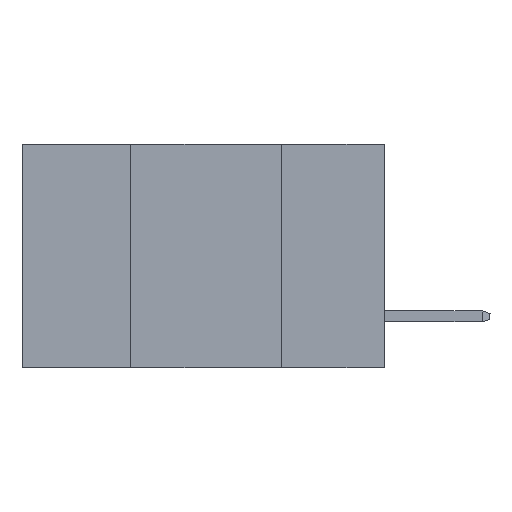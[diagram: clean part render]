
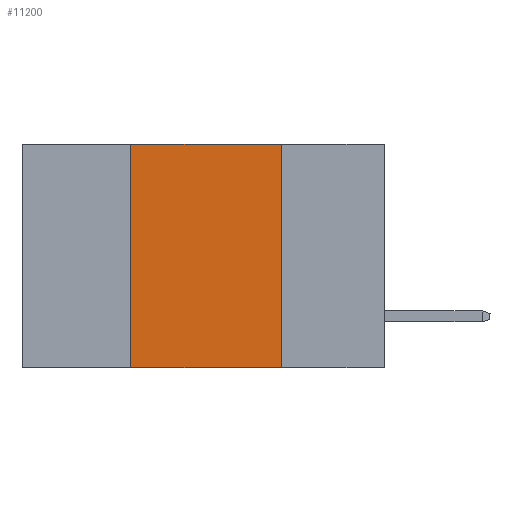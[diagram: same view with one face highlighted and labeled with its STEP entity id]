
A CAD part, left-side view. The second image highlights one B-rep face of the part: STEP entity #11200.
In plain terms, the highlighted planar face has unit normal (-1, 0, 0).
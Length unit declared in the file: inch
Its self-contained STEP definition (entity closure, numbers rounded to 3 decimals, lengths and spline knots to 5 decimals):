
#228 = FACE_OUTER_BOUND ( 'NONE', #8586, .T. ) ;
#1096 = VECTOR ( 'NONE', #9486, 39.37008 ) ;
#1423 = VECTOR ( 'NONE', #8526, 39.37008 ) ;
#1829 = ORIENTED_EDGE ( 'NONE', *, *, #15699, .F. ) ;
#1856 = EDGE_CURVE ( 'NONE', #16244, #8477, #16864, .T. ) ;
#1978 = VERTEX_POINT ( 'NONE', #8205 ) ;
#2695 = CARTESIAN_POINT ( 'NONE',  ( 0., 0.6, -0.37 ) ) ;
#3433 = ORIENTED_EDGE ( 'NONE', *, *, #11694, .F. ) ;
#3590 = CARTESIAN_POINT ( 'NONE',  ( 0., 0.42, -0.37 ) ) ;
#4067 = CARTESIAN_POINT ( 'NONE',  ( 0., 0.42, -0.37 ) ) ;
#4308 = CARTESIAN_POINT ( 'NONE',  ( 0., 0.17, 0. ) ) ;
#4426 = VERTEX_POINT ( 'NONE', #4308 ) ;
#4501 = PLANE ( 'NONE',  #10240 ) ;
#4514 = VECTOR ( 'NONE', #8567, 39.37008 ) ;
#6385 = LINE ( 'NONE', #12284, #13031 ) ;
#8205 = CARTESIAN_POINT ( 'NONE',  ( 0., 0.17, -0.37 ) ) ;
#8477 = VERTEX_POINT ( 'NONE', #18538 ) ;
#8526 = DIRECTION ( 'NONE',  ( 0., -1., 0. ) ) ;
#8567 = DIRECTION ( 'NONE',  ( 0., -1., 0. ) ) ;
#8586 = EDGE_LOOP ( 'NONE', ( #3433, #1829, #9095, #10768 ) ) ;
#9095 = ORIENTED_EDGE ( 'NONE', *, *, #1856, .F. ) ;
#9482 = DIRECTION ( 'NONE',  ( 0., 0., -1. ) ) ;
#9486 = DIRECTION ( 'NONE',  ( 0., 0., 1. ) ) ;
#10240 = AXIS2_PLACEMENT_3D ( 'NONE', #15158, #17869, #10695 ) ;
#10695 = DIRECTION ( 'NONE',  ( 0., 0., -1. ) ) ;
#10768 = ORIENTED_EDGE ( 'NONE', *, *, #18221, .T. ) ;
#11200 = ADVANCED_FACE ( 'NONE', ( #228 ), #4501, .F. ) ;
#11694 = EDGE_CURVE ( 'NONE', #4426, #1978, #6385, .T. ) ;
#11716 = CARTESIAN_POINT ( 'NONE',  ( 0., 0.6, 0. ) ) ;
#12284 = CARTESIAN_POINT ( 'NONE',  ( 0., 0.17, -0.37 ) ) ;
#13031 = VECTOR ( 'NONE', #9482, 39.37008 ) ;
#14496 = LINE ( 'NONE', #2695, #4514 ) ;
#15158 = CARTESIAN_POINT ( 'NONE',  ( 0., 0.6, 0. ) ) ;
#15699 = EDGE_CURVE ( 'NONE', #8477, #4426, #15810, .T. ) ;
#15810 = LINE ( 'NONE', #11716, #1423 ) ;
#16244 = VERTEX_POINT ( 'NONE', #4067 ) ;
#16864 = LINE ( 'NONE', #3590, #1096 ) ;
#17869 = DIRECTION ( 'NONE',  ( 1., 0., 0. ) ) ;
#18221 = EDGE_CURVE ( 'NONE', #16244, #1978, #14496, .T. ) ;
#18538 = CARTESIAN_POINT ( 'NONE',  ( 0., 0.42, 0. ) ) ;
